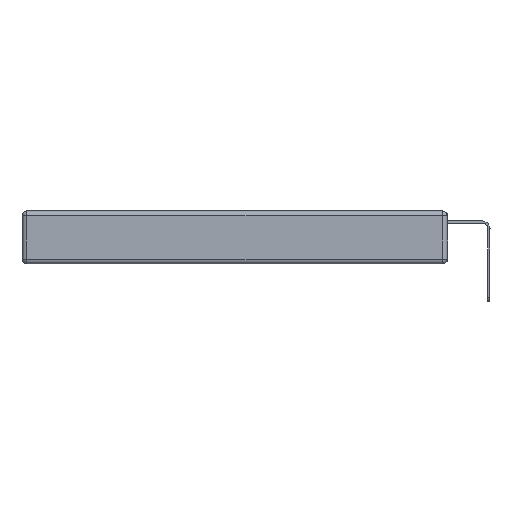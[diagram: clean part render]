
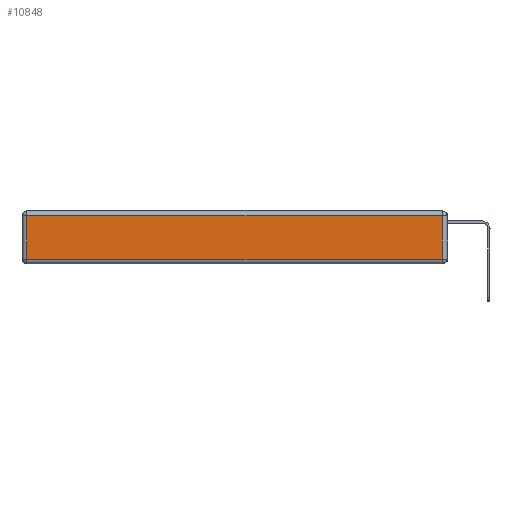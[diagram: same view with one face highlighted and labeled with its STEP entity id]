
A CAD part, left-side view. The second image highlights one B-rep face of the part: STEP entity #10848.
In plain terms, the highlighted planar face has unit normal (-1, 0, 0).
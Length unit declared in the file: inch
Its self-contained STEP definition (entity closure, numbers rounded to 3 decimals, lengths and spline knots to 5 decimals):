
#15 = DIRECTION ( 'NONE',  ( -1., 0., 0. ) ) ;
#141 = VERTEX_POINT ( 'NONE', #10903 ) ;
#1113 = ORIENTED_EDGE ( 'NONE', *, *, #11509, .T. ) ;
#1305 = PLANE ( 'NONE',  #12660 ) ;
#2242 = VECTOR ( 'NONE', #15778, 39.37008 ) ;
#2786 = CARTESIAN_POINT ( 'NONE',  ( 0., 2.72, -0.313 ) ) ;
#3331 = ORIENTED_EDGE ( 'NONE', *, *, #5559, .T. ) ;
#3684 = VECTOR ( 'NONE', #10862, 39.37008 ) ;
#4000 = EDGE_CURVE ( 'NONE', #141, #10484, #15796, .T. ) ;
#5517 = LINE ( 'NONE', #11847, #2242 ) ;
#5553 = VERTEX_POINT ( 'NONE', #10925 ) ;
#5559 = EDGE_CURVE ( 'NONE', #5553, #6901, #15100, .T. ) ;
#6901 = VERTEX_POINT ( 'NONE', #2786 ) ;
#6911 = CARTESIAN_POINT ( 'NONE',  ( 0., 2.72, -0.343 ) ) ;
#7441 = LINE ( 'NONE', #10411, #13162 ) ;
#8011 = EDGE_LOOP ( 'NONE', ( #1113, #10334, #16213, #3331 ) ) ;
#8170 = CARTESIAN_POINT ( 'NONE',  ( 0., 0.03, -0.343 ) ) ;
#8442 = EDGE_CURVE ( 'NONE', #10484, #5553, #7441, .T. ) ;
#9086 = DIRECTION ( 'NONE',  ( 0., 1., 0. ) ) ;
#9620 = DIRECTION ( 'NONE',  ( 0., 0., 1. ) ) ;
#10241 = FACE_OUTER_BOUND ( 'NONE', #8011, .T. ) ;
#10334 = ORIENTED_EDGE ( 'NONE', *, *, #4000, .T. ) ;
#10411 = CARTESIAN_POINT ( 'NONE',  ( 0., 2.75, -0.03 ) ) ;
#10484 = VERTEX_POINT ( 'NONE', #13634 ) ;
#10848 = ADVANCED_FACE ( 'NONE', ( #10241 ), #1305, .T. ) ;
#10862 = DIRECTION ( 'NONE',  ( 0., 0., -1. ) ) ;
#10903 = CARTESIAN_POINT ( 'NONE',  ( 0., 0.03, -0.313 ) ) ;
#10925 = CARTESIAN_POINT ( 'NONE',  ( 0., 2.72, -0.03 ) ) ;
#11509 = EDGE_CURVE ( 'NONE', #6901, #141, #5517, .T. ) ;
#11847 = CARTESIAN_POINT ( 'NONE',  ( 0., 0., -0.313 ) ) ;
#12321 = VECTOR ( 'NONE', #9620, 39.37008 ) ;
#12660 = AXIS2_PLACEMENT_3D ( 'NONE', #13007, #15, #15739 ) ;
#13007 = CARTESIAN_POINT ( 'NONE',  ( 0., 0., -0.343 ) ) ;
#13162 = VECTOR ( 'NONE', #9086, 39.37008 ) ;
#13634 = CARTESIAN_POINT ( 'NONE',  ( 0., 0.03, -0.03 ) ) ;
#15100 = LINE ( 'NONE', #6911, #3684 ) ;
#15739 = DIRECTION ( 'NONE',  ( 0., 0., 1. ) ) ;
#15778 = DIRECTION ( 'NONE',  ( 0., -1., 0. ) ) ;
#15796 = LINE ( 'NONE', #8170, #12321 ) ;
#16213 = ORIENTED_EDGE ( 'NONE', *, *, #8442, .T. ) ;
